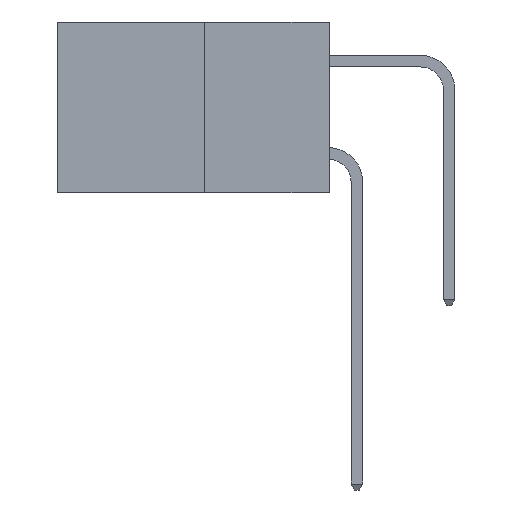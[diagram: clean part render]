
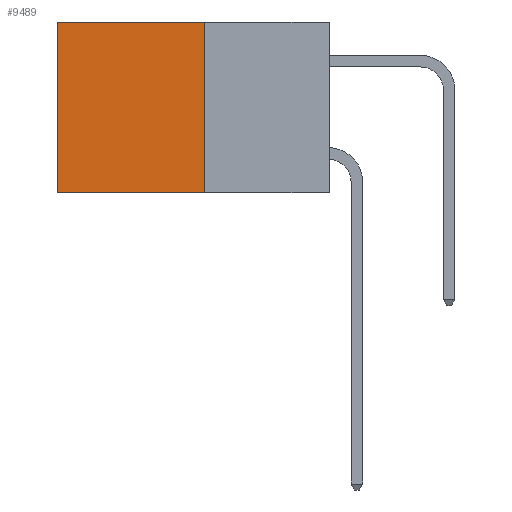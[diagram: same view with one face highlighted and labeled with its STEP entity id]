
A CAD part, left-side view. The second image highlights one B-rep face of the part: STEP entity #9489.
In plain terms, the highlighted planar face has unit normal (-1, 0, 0).
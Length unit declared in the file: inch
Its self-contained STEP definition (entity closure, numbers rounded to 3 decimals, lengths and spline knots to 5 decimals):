
#906 = VERTEX_POINT ( 'NONE', #13314 ) ;
#2317 = EDGE_CURVE ( 'NONE', #5166, #16675, #28199, .T. ) ;
#4103 = ORIENTED_EDGE ( 'NONE', *, *, #2317, .T. ) ;
#4179 = DIRECTION ( 'NONE',  ( 0., 1., 0. ) ) ;
#4670 = VERTEX_POINT ( 'NONE', #20267 ) ;
#5097 = DIRECTION ( 'NONE',  ( 0., 0., -1. ) ) ;
#5166 = VERTEX_POINT ( 'NONE', #9737 ) ;
#5685 = ORIENTED_EDGE ( 'NONE', *, *, #28530, .F. ) ;
#7132 = EDGE_CURVE ( 'NONE', #906, #5166, #16170, .T. ) ;
#7874 = VECTOR ( 'NONE', #14407, 39.37008 ) ;
#8074 = VECTOR ( 'NONE', #5097, 39.37008 ) ;
#9489 = ADVANCED_FACE ( 'NONE', ( #21464 ), #9541, .F. ) ;
#9541 = PLANE ( 'NONE',  #26203 ) ;
#9612 = VECTOR ( 'NONE', #4179, 39.37008 ) ;
#9737 = CARTESIAN_POINT ( 'NONE',  ( 0.277, 0.59, 0. ) ) ;
#11171 = EDGE_LOOP ( 'NONE', ( #4103, #24593, #5685, #18505 ) ) ;
#12025 = CARTESIAN_POINT ( 'NONE',  ( 0.277, 0.27, -0.37 ) ) ;
#12036 = VECTOR ( 'NONE', #12204, 39.37008 ) ;
#12204 = DIRECTION ( 'NONE',  ( 0., 1., 0. ) ) ;
#12791 = LINE ( 'NONE', #24438, #12036 ) ;
#13314 = CARTESIAN_POINT ( 'NONE',  ( 0.277, 0.27, 0. ) ) ;
#14091 = CARTESIAN_POINT ( 'NONE',  ( 0.277, 0.27, 0. ) ) ;
#14407 = DIRECTION ( 'NONE',  ( 0., 0., -1. ) ) ;
#14501 = DIRECTION ( 'NONE',  ( 1., 0., 0. ) ) ;
#15436 = LINE ( 'NONE', #17466, #8074 ) ;
#15797 = CARTESIAN_POINT ( 'NONE',  ( 0.277, 0.59, -0.37 ) ) ;
#16170 = LINE ( 'NONE', #14091, #9612 ) ;
#16584 = CARTESIAN_POINT ( 'NONE',  ( 0.277, 0.59, -0.37 ) ) ;
#16675 = VERTEX_POINT ( 'NONE', #16584 ) ;
#17466 = CARTESIAN_POINT ( 'NONE',  ( 0.277, 0.27, -0.37 ) ) ;
#18505 = ORIENTED_EDGE ( 'NONE', *, *, #7132, .T. ) ;
#20267 = CARTESIAN_POINT ( 'NONE',  ( 0.277, 0.27, -0.37 ) ) ;
#21464 = FACE_OUTER_BOUND ( 'NONE', #11171, .T. ) ;
#24438 = CARTESIAN_POINT ( 'NONE',  ( 0.277, 0.27, -0.37 ) ) ;
#24593 = ORIENTED_EDGE ( 'NONE', *, *, #27518, .F. ) ;
#26203 = AXIS2_PLACEMENT_3D ( 'NONE', #12025, #14501, #31468 ) ;
#27518 = EDGE_CURVE ( 'NONE', #4670, #16675, #12791, .T. ) ;
#28199 = LINE ( 'NONE', #15797, #7874 ) ;
#28530 = EDGE_CURVE ( 'NONE', #906, #4670, #15436, .T. ) ;
#31468 = DIRECTION ( 'NONE',  ( 0., 0., -1. ) ) ;
